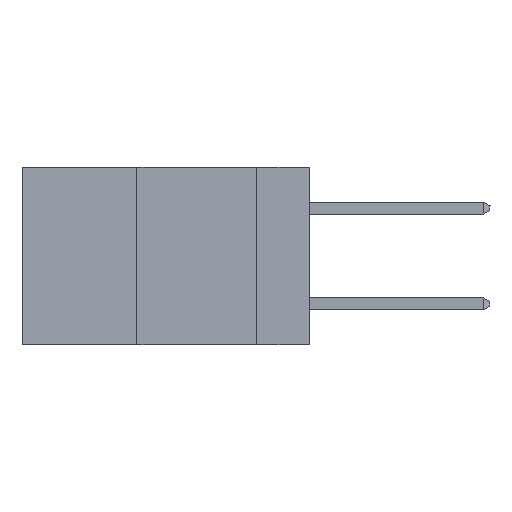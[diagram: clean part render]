
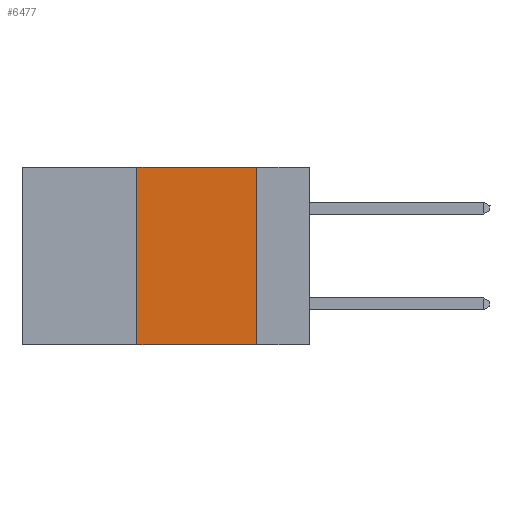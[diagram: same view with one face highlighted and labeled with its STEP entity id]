
A CAD part, left-side view. The second image highlights one B-rep face of the part: STEP entity #6477.
In plain terms, the highlighted planar face has unit normal (-1, 0, 0).
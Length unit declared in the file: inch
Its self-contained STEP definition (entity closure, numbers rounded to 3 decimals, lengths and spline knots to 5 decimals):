
#441 = CARTESIAN_POINT ( 'NONE',  ( 0., 0.6, 0. ) ) ;
#560 = VECTOR ( 'NONE', #5946, 39.37008 ) ;
#1156 = DIRECTION ( 'NONE',  ( 0., 0., -1. ) ) ;
#1461 = ORIENTED_EDGE ( 'NONE', *, *, #12811, .F. ) ;
#1628 = CARTESIAN_POINT ( 'NONE',  ( 0., 0.36, 0. ) ) ;
#2030 = VERTEX_POINT ( 'NONE', #9211 ) ;
#2597 = VECTOR ( 'NONE', #4786, 39.37008 ) ;
#2708 = EDGE_CURVE ( 'NONE', #2030, #13575, #9689, .T. ) ;
#2771 = ORIENTED_EDGE ( 'NONE', *, *, #13701, .F. ) ;
#2907 = CARTESIAN_POINT ( 'NONE',  ( 0., 0.6, -0.37 ) ) ;
#2959 = ORIENTED_EDGE ( 'NONE', *, *, #6099, .T. ) ;
#3101 = CARTESIAN_POINT ( 'NONE',  ( 0., 0.36, -0.37 ) ) ;
#3273 = CARTESIAN_POINT ( 'NONE',  ( 0., 0.11, -0.37 ) ) ;
#3380 = DIRECTION ( 'NONE',  ( 0., 0., -1. ) ) ;
#3611 = ORIENTED_EDGE ( 'NONE', *, *, #2708, .F. ) ;
#4649 = LINE ( 'NONE', #441, #2597 ) ;
#4786 = DIRECTION ( 'NONE',  ( 0., -1., 0. ) ) ;
#5021 = AXIS2_PLACEMENT_3D ( 'NONE', #12833, #10838, #3380 ) ;
#5440 = FACE_OUTER_BOUND ( 'NONE', #13523, .T. ) ;
#5946 = DIRECTION ( 'NONE',  ( 0., 0., 1. ) ) ;
#6099 = EDGE_CURVE ( 'NONE', #9450, #13575, #11721, .T. ) ;
#6477 = ADVANCED_FACE ( 'NONE', ( #5440 ), #7435, .F. ) ;
#7435 = PLANE ( 'NONE',  #5021 ) ;
#8408 = VECTOR ( 'NONE', #11575, 39.37008 ) ;
#8480 = VERTEX_POINT ( 'NONE', #11100 ) ;
#9211 = CARTESIAN_POINT ( 'NONE',  ( 0., 0.11, 0. ) ) ;
#9450 = VERTEX_POINT ( 'NONE', #3101 ) ;
#9689 = LINE ( 'NONE', #9959, #11192 ) ;
#9959 = CARTESIAN_POINT ( 'NONE',  ( 0., 0.11, 0. ) ) ;
#10838 = DIRECTION ( 'NONE',  ( 1., 0., 0. ) ) ;
#11100 = CARTESIAN_POINT ( 'NONE',  ( 0., 0.36, 0. ) ) ;
#11192 = VECTOR ( 'NONE', #1156, 39.37008 ) ;
#11344 = LINE ( 'NONE', #1628, #560 ) ;
#11575 = DIRECTION ( 'NONE',  ( 0., -1., 0. ) ) ;
#11721 = LINE ( 'NONE', #2907, #8408 ) ;
#12811 = EDGE_CURVE ( 'NONE', #8480, #2030, #4649, .T. ) ;
#12833 = CARTESIAN_POINT ( 'NONE',  ( 0., 0.6, 0. ) ) ;
#13523 = EDGE_LOOP ( 'NONE', ( #3611, #1461, #2771, #2959 ) ) ;
#13575 = VERTEX_POINT ( 'NONE', #3273 ) ;
#13701 = EDGE_CURVE ( 'NONE', #9450, #8480, #11344, .T. ) ;
